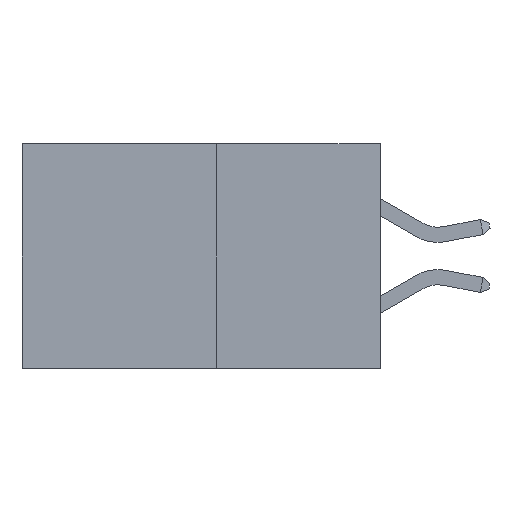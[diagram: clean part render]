
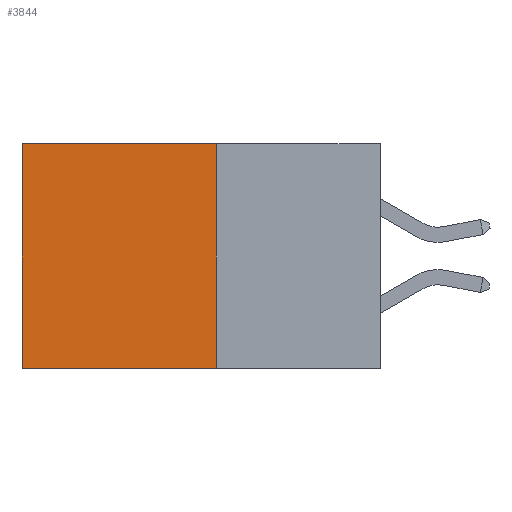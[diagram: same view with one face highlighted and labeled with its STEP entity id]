
A CAD part, left-side view. The second image highlights one B-rep face of the part: STEP entity #3844.
In plain terms, the highlighted planar face has unit normal (-1, 0, 0).
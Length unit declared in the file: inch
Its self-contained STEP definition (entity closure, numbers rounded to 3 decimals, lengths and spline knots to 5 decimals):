
#823 = DIRECTION ( 'NONE',  ( 1., 0., 0. ) ) ;
#3377 = CARTESIAN_POINT ( 'NONE',  ( 0.277, 0.27, -0.37 ) ) ;
#3838 = CARTESIAN_POINT ( 'NONE',  ( 0.277, 0.59, -0.37 ) ) ;
#3844 = ADVANCED_FACE ( 'NONE', ( #16752 ), #16524, .F. ) ;
#4731 = LINE ( 'NONE', #3838, #10868 ) ;
#7674 = LINE ( 'NONE', #10002, #27794 ) ;
#8443 = ORIENTED_EDGE ( 'NONE', *, *, #10017, .T. ) ;
#9236 = DIRECTION ( 'NONE',  ( 0., 0., -1. ) ) ;
#9819 = VERTEX_POINT ( 'NONE', #16274 ) ;
#10002 = CARTESIAN_POINT ( 'NONE',  ( 0.277, 0.27, -0.37 ) ) ;
#10017 = EDGE_CURVE ( 'NONE', #12732, #9819, #4731, .T. ) ;
#10440 = EDGE_CURVE ( 'NONE', #33125, #18904, #27372, .T. ) ;
#10868 = VECTOR ( 'NONE', #9236, 39.37008 ) ;
#12732 = VERTEX_POINT ( 'NONE', #25072 ) ;
#14050 = EDGE_CURVE ( 'NONE', #33125, #12732, #16718, .T. ) ;
#14957 = AXIS2_PLACEMENT_3D ( 'NONE', #27076, #823, #19191 ) ;
#16274 = CARTESIAN_POINT ( 'NONE',  ( 0.277, 0.59, -0.37 ) ) ;
#16524 = PLANE ( 'NONE',  #14957 ) ;
#16718 = LINE ( 'NONE', #24595, #30772 ) ;
#16752 = FACE_OUTER_BOUND ( 'NONE', #31628, .T. ) ;
#18904 = VERTEX_POINT ( 'NONE', #3377 ) ;
#19191 = DIRECTION ( 'NONE',  ( 0., 0., -1. ) ) ;
#21237 = DIRECTION ( 'NONE',  ( 0., 0., -1. ) ) ;
#21771 = ORIENTED_EDGE ( 'NONE', *, *, #14050, .T. ) ;
#22543 = CARTESIAN_POINT ( 'NONE',  ( 0.277, 0.27, 0. ) ) ;
#22981 = EDGE_CURVE ( 'NONE', #18904, #9819, #7674, .T. ) ;
#24595 = CARTESIAN_POINT ( 'NONE',  ( 0.277, 0.27, 0. ) ) ;
#25072 = CARTESIAN_POINT ( 'NONE',  ( 0.277, 0.59, 0. ) ) ;
#26065 = ORIENTED_EDGE ( 'NONE', *, *, #22981, .F. ) ;
#26558 = CARTESIAN_POINT ( 'NONE',  ( 0.277, 0.27, -0.37 ) ) ;
#27076 = CARTESIAN_POINT ( 'NONE',  ( 0.277, 0.27, -0.37 ) ) ;
#27372 = LINE ( 'NONE', #26558, #28209 ) ;
#27794 = VECTOR ( 'NONE', #28380, 39.37008 ) ;
#28209 = VECTOR ( 'NONE', #21237, 39.37008 ) ;
#28380 = DIRECTION ( 'NONE',  ( 0., 1., 0. ) ) ;
#29934 = ORIENTED_EDGE ( 'NONE', *, *, #10440, .F. ) ;
#30772 = VECTOR ( 'NONE', #32301, 39.37008 ) ;
#31628 = EDGE_LOOP ( 'NONE', ( #8443, #26065, #29934, #21771 ) ) ;
#32301 = DIRECTION ( 'NONE',  ( 0., 1., 0. ) ) ;
#33125 = VERTEX_POINT ( 'NONE', #22543 ) ;
